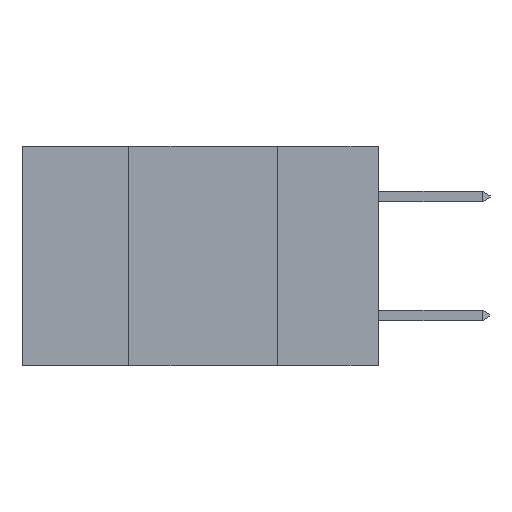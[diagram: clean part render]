
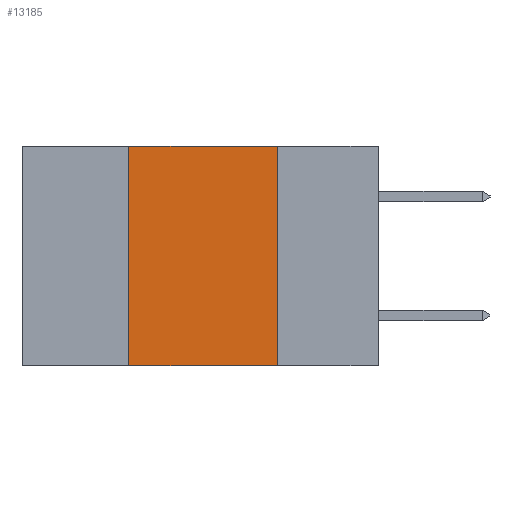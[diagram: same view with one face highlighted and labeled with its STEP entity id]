
A CAD part, left-side view. The second image highlights one B-rep face of the part: STEP entity #13185.
In plain terms, the highlighted planar face has unit normal (-1, 0, 0).
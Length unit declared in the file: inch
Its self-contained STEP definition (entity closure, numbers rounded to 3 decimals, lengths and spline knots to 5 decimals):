
#82 = ORIENTED_EDGE ( 'NONE', *, *, #22434, .F. ) ;
#734 = LINE ( 'NONE', #6886, #18814 ) ;
#1180 = VERTEX_POINT ( 'NONE', #14248 ) ;
#1448 = VERTEX_POINT ( 'NONE', #9519 ) ;
#1961 = VERTEX_POINT ( 'NONE', #13490 ) ;
#3257 = CARTESIAN_POINT ( 'NONE',  ( 0., 0.42, 0. ) ) ;
#6399 = CARTESIAN_POINT ( 'NONE',  ( 0., 0.42, -0.37 ) ) ;
#6886 = CARTESIAN_POINT ( 'NONE',  ( 0., 0.6, 0. ) ) ;
#8467 = ORIENTED_EDGE ( 'NONE', *, *, #21265, .F. ) ;
#8616 = VECTOR ( 'NONE', #19577, 39.37008 ) ;
#9519 = CARTESIAN_POINT ( 'NONE',  ( 0., 0.17, -0.37 ) ) ;
#10313 = FACE_OUTER_BOUND ( 'NONE', #10538, .T. ) ;
#10493 = DIRECTION ( 'NONE',  ( 0., 0., -1. ) ) ;
#10538 = EDGE_LOOP ( 'NONE', ( #8467, #82, #14696, #11189 ) ) ;
#10862 = EDGE_CURVE ( 'NONE', #1961, #1448, #19714, .T. ) ;
#11009 = CARTESIAN_POINT ( 'NONE',  ( 0., 0.17, -0.37 ) ) ;
#11189 = ORIENTED_EDGE ( 'NONE', *, *, #10862, .T. ) ;
#11604 = LINE ( 'NONE', #11009, #8616 ) ;
#11891 = VERTEX_POINT ( 'NONE', #3257 ) ;
#12105 = VECTOR ( 'NONE', #21982, 39.37008 ) ;
#12683 = AXIS2_PLACEMENT_3D ( 'NONE', #19080, #20836, #10493 ) ;
#13007 = DIRECTION ( 'NONE',  ( 0., -1., 0. ) ) ;
#13185 = ADVANCED_FACE ( 'NONE', ( #10313 ), #15630, .F. ) ;
#13490 = CARTESIAN_POINT ( 'NONE',  ( 0., 0.42, -0.37 ) ) ;
#14248 = CARTESIAN_POINT ( 'NONE',  ( 0., 0.17, 0. ) ) ;
#14696 = ORIENTED_EDGE ( 'NONE', *, *, #15484, .F. ) ;
#15484 = EDGE_CURVE ( 'NONE', #1961, #11891, #21292, .T. ) ;
#15630 = PLANE ( 'NONE',  #12683 ) ;
#18814 = VECTOR ( 'NONE', #22452, 39.37008 ) ;
#19080 = CARTESIAN_POINT ( 'NONE',  ( 0., 0.6, 0. ) ) ;
#19577 = DIRECTION ( 'NONE',  ( 0., 0., -1. ) ) ;
#19714 = LINE ( 'NONE', #19837, #20264 ) ;
#19837 = CARTESIAN_POINT ( 'NONE',  ( 0., 0.6, -0.37 ) ) ;
#20264 = VECTOR ( 'NONE', #13007, 39.37008 ) ;
#20836 = DIRECTION ( 'NONE',  ( 1., 0., 0. ) ) ;
#21265 = EDGE_CURVE ( 'NONE', #1180, #1448, #11604, .T. ) ;
#21292 = LINE ( 'NONE', #6399, #12105 ) ;
#21982 = DIRECTION ( 'NONE',  ( 0., 0., 1. ) ) ;
#22434 = EDGE_CURVE ( 'NONE', #11891, #1180, #734, .T. ) ;
#22452 = DIRECTION ( 'NONE',  ( 0., -1., 0. ) ) ;
